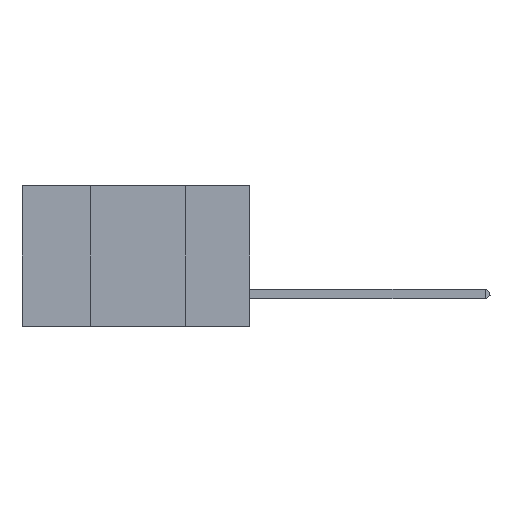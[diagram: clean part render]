
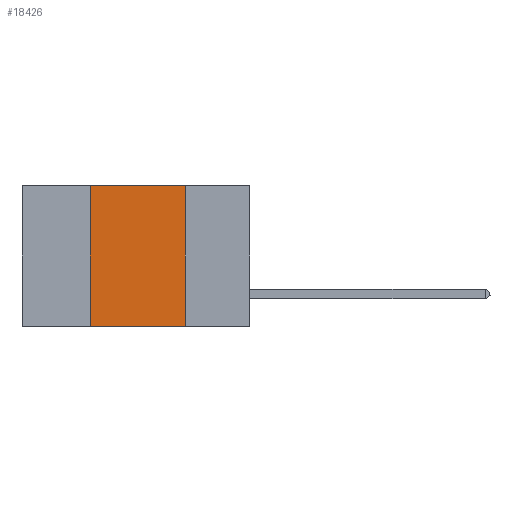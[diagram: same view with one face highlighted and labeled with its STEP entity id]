
A CAD part, left-side view. The second image highlights one B-rep face of the part: STEP entity #18426.
In plain terms, the highlighted planar face has unit normal (-1, 0, 0).
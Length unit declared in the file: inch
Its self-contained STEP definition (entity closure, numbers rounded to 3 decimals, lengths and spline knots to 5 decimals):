
#3450 = ORIENTED_EDGE ( 'NONE', *, *, #44766, .T. ) ;
#7825 = LINE ( 'NONE', #34030, #13276 ) ;
#10083 = VECTOR ( 'NONE', #23420, 39.37008 ) ;
#10795 = EDGE_CURVE ( 'NONE', #21348, #42001, #34749, .T. ) ;
#13276 = VECTOR ( 'NONE', #20120, 39.37008 ) ;
#13455 = FACE_OUTER_BOUND ( 'NONE', #30780, .T. ) ;
#13965 = VECTOR ( 'NONE', #37848, 39.37008 ) ;
#14476 = DIRECTION ( 'NONE',  ( 1., 0., 0. ) ) ;
#14857 = AXIS2_PLACEMENT_3D ( 'NONE', #32107, #14476, #18156 ) ;
#16772 = CARTESIAN_POINT ( 'NONE',  ( 0., 0.17, 0. ) ) ;
#17156 = VECTOR ( 'NONE', #37021, 39.37008 ) ;
#17788 = LINE ( 'NONE', #34337, #13965 ) ;
#18156 = DIRECTION ( 'NONE',  ( 0., 0., -1. ) ) ;
#18426 = ADVANCED_FACE ( 'NONE', ( #13455 ), #21398, .F. ) ;
#18662 = VERTEX_POINT ( 'NONE', #19216 ) ;
#19216 = CARTESIAN_POINT ( 'NONE',  ( 0., 0.17, -0.37 ) ) ;
#19844 = ORIENTED_EDGE ( 'NONE', *, *, #10795, .F. ) ;
#20120 = DIRECTION ( 'NONE',  ( 0., -1., 0. ) ) ;
#20942 = CARTESIAN_POINT ( 'NONE',  ( 0., 0.42, 0. ) ) ;
#21348 = VERTEX_POINT ( 'NONE', #20942 ) ;
#21398 = PLANE ( 'NONE',  #14857 ) ;
#22701 = ORIENTED_EDGE ( 'NONE', *, *, #28869, .F. ) ;
#23420 = DIRECTION ( 'NONE',  ( 0., -1., 0. ) ) ;
#25649 = ORIENTED_EDGE ( 'NONE', *, *, #42937, .F. ) ;
#27656 = CARTESIAN_POINT ( 'NONE',  ( 0., 0.42, -0.37 ) ) ;
#28869 = EDGE_CURVE ( 'NONE', #42001, #18662, #36352, .T. ) ;
#29049 = VERTEX_POINT ( 'NONE', #27656 ) ;
#30780 = EDGE_LOOP ( 'NONE', ( #22701, #19844, #25649, #3450 ) ) ;
#32107 = CARTESIAN_POINT ( 'NONE',  ( 0., 0.6, 0. ) ) ;
#34030 = CARTESIAN_POINT ( 'NONE',  ( 0., 0.6, -0.37 ) ) ;
#34337 = CARTESIAN_POINT ( 'NONE',  ( 0., 0.42, 0. ) ) ;
#34749 = LINE ( 'NONE', #44509, #10083 ) ;
#36352 = LINE ( 'NONE', #44620, #17156 ) ;
#37021 = DIRECTION ( 'NONE',  ( 0., 0., -1. ) ) ;
#37848 = DIRECTION ( 'NONE',  ( 0., 0., 1. ) ) ;
#42001 = VERTEX_POINT ( 'NONE', #16772 ) ;
#42937 = EDGE_CURVE ( 'NONE', #29049, #21348, #17788, .T. ) ;
#44509 = CARTESIAN_POINT ( 'NONE',  ( 0., 0.6, 0. ) ) ;
#44620 = CARTESIAN_POINT ( 'NONE',  ( 0., 0.17, 0. ) ) ;
#44766 = EDGE_CURVE ( 'NONE', #29049, #18662, #7825, .T. ) ;
